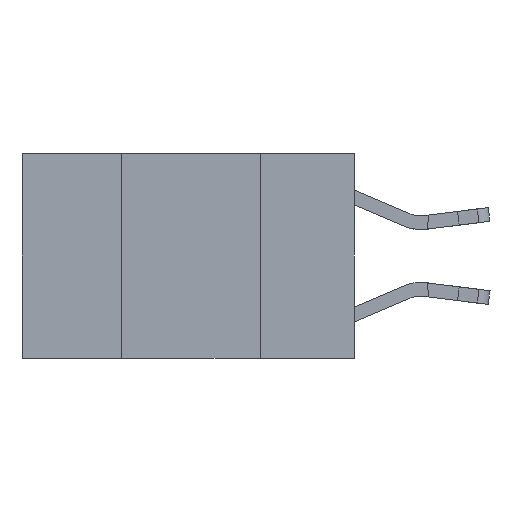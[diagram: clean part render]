
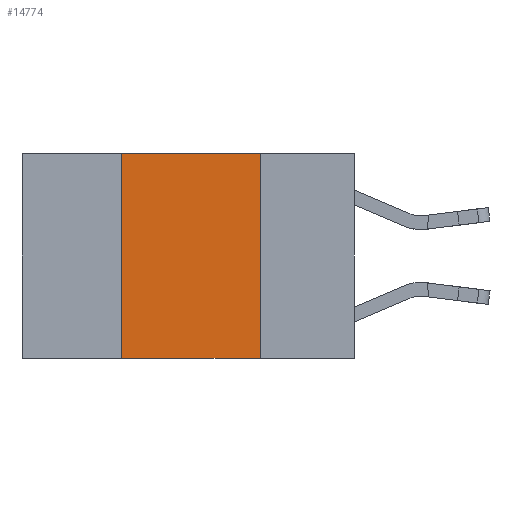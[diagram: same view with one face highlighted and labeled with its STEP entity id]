
A CAD part, left-side view. The second image highlights one B-rep face of the part: STEP entity #14774.
In plain terms, the highlighted planar face has unit normal (-1, 0, 0).
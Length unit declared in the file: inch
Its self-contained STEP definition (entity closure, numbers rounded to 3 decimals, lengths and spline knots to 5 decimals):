
#2119 = VECTOR ( 'NONE', #5916, 39.37008 ) ;
#3060 = CARTESIAN_POINT ( 'NONE',  ( 0., 0.17, 0. ) ) ;
#3214 = CARTESIAN_POINT ( 'NONE',  ( 0., 0.17, -0.37 ) ) ;
#3761 = EDGE_CURVE ( 'NONE', #7373, #8942, #25896, .T. ) ;
#4881 = AXIS2_PLACEMENT_3D ( 'NONE', #11092, #25675, #13222 ) ;
#5687 = DIRECTION ( 'NONE',  ( 0., -1., 0. ) ) ;
#5916 = DIRECTION ( 'NONE',  ( 0., -1., 0. ) ) ;
#6727 = ORIENTED_EDGE ( 'NONE', *, *, #9351, .F. ) ;
#7373 = VERTEX_POINT ( 'NONE', #21954 ) ;
#8942 = VERTEX_POINT ( 'NONE', #3214 ) ;
#9351 = EDGE_CURVE ( 'NONE', #26060, #11436, #22174, .T. ) ;
#9676 = CARTESIAN_POINT ( 'NONE',  ( 0., 0.42, -0.37 ) ) ;
#11092 = CARTESIAN_POINT ( 'NONE',  ( 0., 0.6, 0. ) ) ;
#11436 = VERTEX_POINT ( 'NONE', #14860 ) ;
#12131 = CARTESIAN_POINT ( 'NONE',  ( 0., 0.6, -0.37 ) ) ;
#13222 = DIRECTION ( 'NONE',  ( 0., 0., -1. ) ) ;
#13915 = LINE ( 'NONE', #12131, #2119 ) ;
#14019 = CARTESIAN_POINT ( 'NONE',  ( 0., 0.6, 0. ) ) ;
#14774 = ADVANCED_FACE ( 'NONE', ( #15406 ), #21475, .F. ) ;
#14860 = CARTESIAN_POINT ( 'NONE',  ( 0., 0.42, 0. ) ) ;
#14923 = CARTESIAN_POINT ( 'NONE',  ( 0., 0.42, 0. ) ) ;
#15402 = EDGE_LOOP ( 'NONE', ( #25674, #20498, #6727, #23603 ) ) ;
#15406 = FACE_OUTER_BOUND ( 'NONE', #15402, .T. ) ;
#15486 = VECTOR ( 'NONE', #26033, 39.37008 ) ;
#17281 = VECTOR ( 'NONE', #23278, 39.37008 ) ;
#18284 = VECTOR ( 'NONE', #5687, 39.37008 ) ;
#20498 = ORIENTED_EDGE ( 'NONE', *, *, #23413, .F. ) ;
#21251 = EDGE_CURVE ( 'NONE', #26060, #8942, #13915, .T. ) ;
#21475 = PLANE ( 'NONE',  #4881 ) ;
#21954 = CARTESIAN_POINT ( 'NONE',  ( 0., 0.17, 0. ) ) ;
#22174 = LINE ( 'NONE', #14923, #17281 ) ;
#23278 = DIRECTION ( 'NONE',  ( 0., 0., 1. ) ) ;
#23413 = EDGE_CURVE ( 'NONE', #11436, #7373, #23837, .T. ) ;
#23603 = ORIENTED_EDGE ( 'NONE', *, *, #21251, .T. ) ;
#23837 = LINE ( 'NONE', #14019, #18284 ) ;
#25674 = ORIENTED_EDGE ( 'NONE', *, *, #3761, .F. ) ;
#25675 = DIRECTION ( 'NONE',  ( 1., 0., 0. ) ) ;
#25896 = LINE ( 'NONE', #3060, #15486 ) ;
#26033 = DIRECTION ( 'NONE',  ( 0., 0., -1. ) ) ;
#26060 = VERTEX_POINT ( 'NONE', #9676 ) ;
